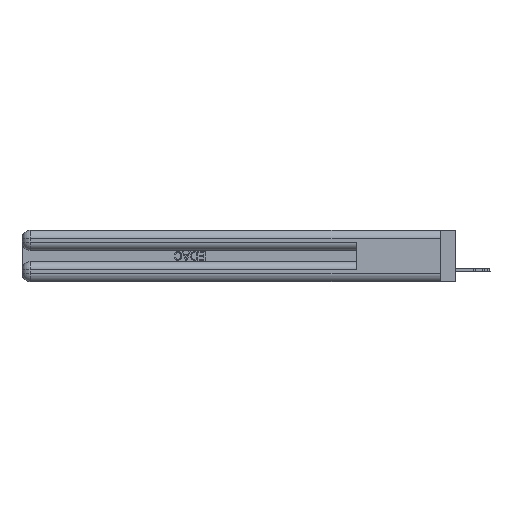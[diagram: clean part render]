
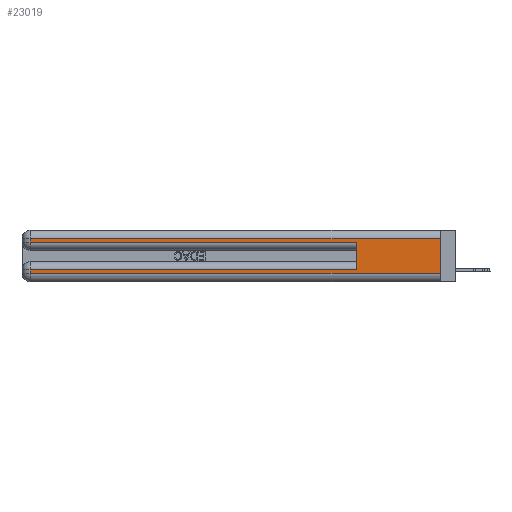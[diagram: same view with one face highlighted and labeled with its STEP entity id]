
A CAD part, left-side view. The second image highlights one B-rep face of the part: STEP entity #23019.
In plain terms, the highlighted planar face has unit normal (-1, 0, 0).
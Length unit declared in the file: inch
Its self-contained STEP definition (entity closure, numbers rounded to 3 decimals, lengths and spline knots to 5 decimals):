
#76 = DIRECTION ( 'NONE',  ( 0., 1., 0. ) ) ;
#100 = CARTESIAN_POINT ( 'NONE',  ( 0., 0.6, 0.085 ) ) ;
#253 = VERTEX_POINT ( 'NONE', #39049 ) ;
#724 = ORIENTED_EDGE ( 'NONE', *, *, #22593, .T. ) ;
#1524 = VECTOR ( 'NONE', #4690, 39.37008 ) ;
#2292 = PLANE ( 'NONE',  #30204 ) ;
#2902 = CARTESIAN_POINT ( 'NONE',  ( 0., 0., 0.37 ) ) ;
#3147 = VECTOR ( 'NONE', #3972, 39.37008 ) ;
#3972 = DIRECTION ( 'NONE',  ( 0., -1., 0. ) ) ;
#4690 = DIRECTION ( 'NONE',  ( 0., 0., -1. ) ) ;
#5293 = CARTESIAN_POINT ( 'NONE',  ( 0., 0., 0.285 ) ) ;
#5474 = ORIENTED_EDGE ( 'NONE', *, *, #39013, .T. ) ;
#7157 = CARTESIAN_POINT ( 'NONE',  ( 0., 2.94, 0.285 ) ) ;
#7294 = LINE ( 'NONE', #5293, #35558 ) ;
#7749 = EDGE_CURVE ( 'NONE', #253, #16617, #21245, .T. ) ;
#8500 = CARTESIAN_POINT ( 'NONE',  ( 0., 0.6, 0.145 ) ) ;
#9862 = CARTESIAN_POINT ( 'NONE',  ( 0., 0.6, 0.285 ) ) ;
#10160 = CARTESIAN_POINT ( 'NONE',  ( 0., 2.94, 0.37 ) ) ;
#10180 = LINE ( 'NONE', #8500, #17200 ) ;
#11166 = CARTESIAN_POINT ( 'NONE',  ( 0., 2.94, 0.31 ) ) ;
#11402 = LINE ( 'NONE', #32164, #28558 ) ;
#11733 = EDGE_CURVE ( 'NONE', #18116, #41777, #7294, .T. ) ;
#12337 = ORIENTED_EDGE ( 'NONE', *, *, #16017, .F. ) ;
#12446 = CARTESIAN_POINT ( 'NONE',  ( 0., 2.94, 0.085 ) ) ;
#13089 = DIRECTION ( 'NONE',  ( 0., 0., -1. ) ) ;
#16017 = EDGE_CURVE ( 'NONE', #29488, #41777, #10180, .T. ) ;
#16617 = VERTEX_POINT ( 'NONE', #32318 ) ;
#16982 = LINE ( 'NONE', #2902, #25568 ) ;
#17200 = VECTOR ( 'NONE', #17455, 39.37008 ) ;
#17455 = DIRECTION ( 'NONE',  ( 0., 0., 1. ) ) ;
#17879 = VERTEX_POINT ( 'NONE', #11166 ) ;
#18116 = VERTEX_POINT ( 'NONE', #7157 ) ;
#18527 = CARTESIAN_POINT ( 'NONE',  ( 0., 0., 0.31 ) ) ;
#18644 = VERTEX_POINT ( 'NONE', #38632 ) ;
#19466 = ORIENTED_EDGE ( 'NONE', *, *, #30015, .F. ) ;
#19676 = LINE ( 'NONE', #18527, #23188 ) ;
#21188 = LINE ( 'NONE', #10160, #28761 ) ;
#21245 = LINE ( 'NONE', #26589, #3147 ) ;
#22151 = ORIENTED_EDGE ( 'NONE', *, *, #36108, .T. ) ;
#22593 = EDGE_CURVE ( 'NONE', #30021, #253, #21188, .T. ) ;
#22757 = EDGE_CURVE ( 'NONE', #17879, #18116, #25165, .T. ) ;
#23019 = ADVANCED_FACE ( 'NONE', ( #35808 ), #2292, .F. ) ;
#23188 = VECTOR ( 'NONE', #37824, 39.37008 ) ;
#25165 = LINE ( 'NONE', #30450, #1524 ) ;
#25568 = VECTOR ( 'NONE', #31450, 39.37008 ) ;
#26589 = CARTESIAN_POINT ( 'NONE',  ( 0., 0., 0.06 ) ) ;
#27784 = ORIENTED_EDGE ( 'NONE', *, *, #7749, .T. ) ;
#28558 = VECTOR ( 'NONE', #76, 39.37008 ) ;
#28761 = VECTOR ( 'NONE', #13089, 39.37008 ) ;
#29488 = VERTEX_POINT ( 'NONE', #100 ) ;
#30015 = EDGE_CURVE ( 'NONE', #18644, #16617, #16982, .T. ) ;
#30021 = VERTEX_POINT ( 'NONE', #12446 ) ;
#30115 = DIRECTION ( 'NONE',  ( 0., -1., 0. ) ) ;
#30204 = AXIS2_PLACEMENT_3D ( 'NONE', #37575, #37431, #34110 ) ;
#30450 = CARTESIAN_POINT ( 'NONE',  ( 0., 2.94, 0.37 ) ) ;
#31450 = DIRECTION ( 'NONE',  ( 0., 0., -1. ) ) ;
#32164 = CARTESIAN_POINT ( 'NONE',  ( 0., 0., 0.085 ) ) ;
#32318 = CARTESIAN_POINT ( 'NONE',  ( 0., 0., 0.06 ) ) ;
#33179 = ORIENTED_EDGE ( 'NONE', *, *, #11733, .T. ) ;
#34110 = DIRECTION ( 'NONE',  ( 0., 0., -1. ) ) ;
#35558 = VECTOR ( 'NONE', #30115, 39.37008 ) ;
#35808 = FACE_OUTER_BOUND ( 'NONE', #40008, .T. ) ;
#36108 = EDGE_CURVE ( 'NONE', #18644, #17879, #19676, .T. ) ;
#36986 = ORIENTED_EDGE ( 'NONE', *, *, #22757, .T. ) ;
#37431 = DIRECTION ( 'NONE',  ( 1., 0., 0. ) ) ;
#37575 = CARTESIAN_POINT ( 'NONE',  ( 0., 0., 0.37 ) ) ;
#37824 = DIRECTION ( 'NONE',  ( 0., 1., 0. ) ) ;
#38632 = CARTESIAN_POINT ( 'NONE',  ( 0., 0., 0.31 ) ) ;
#39013 = EDGE_CURVE ( 'NONE', #29488, #30021, #11402, .T. ) ;
#39049 = CARTESIAN_POINT ( 'NONE',  ( 0., 2.94, 0.06 ) ) ;
#40008 = EDGE_LOOP ( 'NONE', ( #19466, #22151, #36986, #33179, #12337, #5474, #724, #27784 ) ) ;
#41777 = VERTEX_POINT ( 'NONE', #9862 ) ;
